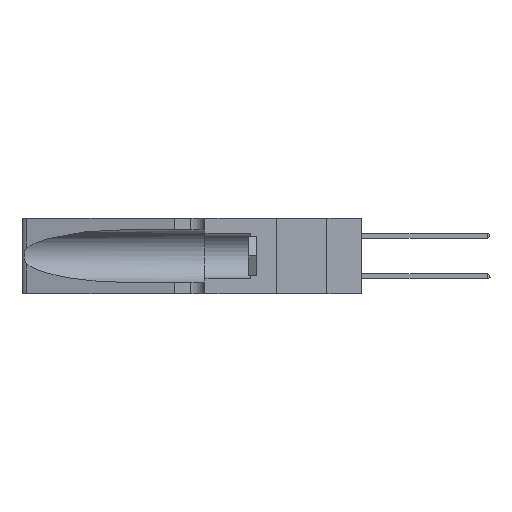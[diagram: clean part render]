
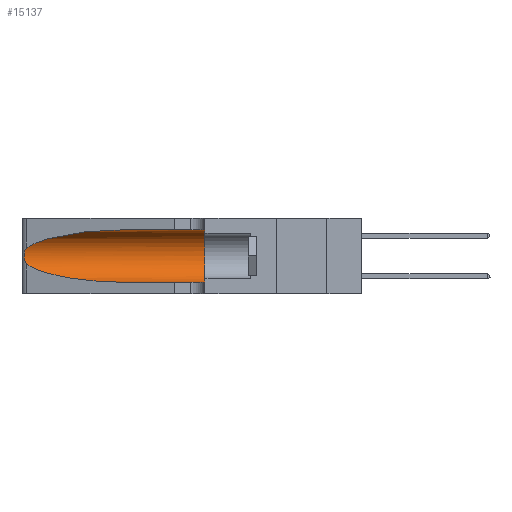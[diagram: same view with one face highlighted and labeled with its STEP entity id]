
A CAD part, left-side view. The second image highlights one B-rep face of the part: STEP entity #15137.
In plain terms, the highlighted cylindrical face has radius 3.308 mm (diameter 6.617 mm), a partial arc.
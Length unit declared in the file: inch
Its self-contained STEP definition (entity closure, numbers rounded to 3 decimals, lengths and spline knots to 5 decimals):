
#39 = CARTESIAN_POINT ( 'NONE',  ( 0.26017, 1.23833, 0.17102 ) ) ;
#55 = ORIENTED_EDGE ( 'NONE', *, *, #19286, .T. ) ;
#152 = CARTESIAN_POINT ( 'NONE',  ( 0.26075, 1.23896, 0.19203 ) ) ;
#261 = CARTESIAN_POINT ( 'NONE',  ( 0.1305, 1.61858, 0.05475 ) ) ;
#587 = CARTESIAN_POINT ( 'NONE',  ( 0.1305, 0.35, 0.185 ) ) ;
#1008 = CARTESIAN_POINT ( 'NONE',  ( 0.25487, 1.22718, 0.22369 ) ) ;
#2813 = CARTESIAN_POINT ( 'NONE',  ( 0.18966, 0.96281, 0.31525 ) ) ;
#3195 = CARTESIAN_POINT ( 'NONE',  ( 0.25639, 1.23186, 0.15144 ) ) ;
#3668 = B_SPLINE_CURVE_WITH_KNOTS ( 'NONE', 3,
 ( #23831, #9269, #23954, #18016, #5847, #26988, #152, #15075, #39, #33325, #36164, #3195, #8902, #30044 ),
 .UNSPECIFIED., .F., .F.,
 ( 4, 2, 2, 2, 2, 2, 4 ),
 ( 0., 0.00027, 0.00053, 0.00107, 0.0016, 0.00187, 0.00214 ),
 .UNSPECIFIED. ) ;
#4745 = VERTEX_POINT ( 'NONE', #27043 ) ;
#5590 = ORIENTED_EDGE ( 'NONE', *, *, #26484, .T. ) ;
#5693 = CARTESIAN_POINT ( 'NONE',  ( 0.1305, 0.72297, 0.31525 ) ) ;
#5847 = CARTESIAN_POINT ( 'NONE',  ( 0.25854, 1.2359, 0.20912 ) ) ;
#5869 =( BOUNDED_CURVE ( )  B_SPLINE_CURVE ( 3, ( #38904, #24022, #11846, #33018 ),
 .UNSPECIFIED., .F., .T. ) 
 B_SPLINE_CURVE_WITH_KNOTS ( ( 4, 4 ),
 ( 3.44316, 4.71239 ),
 .UNSPECIFIED. ) 
 CURVE ( )  GEOMETRIC_REPRESENTATION_ITEM ( )  RATIONAL_B_SPLINE_CURVE ( ( 1., 0.87, 0.87, 1. ) ) 
 REPRESENTATION_ITEM ( '' )  );
#6136 = ORIENTED_EDGE ( 'NONE', *, *, #13346, .T. ) ;
#7118 = VERTEX_POINT ( 'NONE', #35949 ) ;
#7136 = CARTESIAN_POINT ( 'NONE',  ( 0.1305, 0.72297, 0.05475 ) ) ;
#7799 = VERTEX_POINT ( 'NONE', #35772 ) ;
#8902 = CARTESIAN_POINT ( 'NONE',  ( 0.25555, 1.22993, 0.14849 ) ) ;
#9269 = CARTESIAN_POINT ( 'NONE',  ( 0.25555, 1.22994, 0.2215 ) ) ;
#10227 = EDGE_LOOP ( 'NONE', ( #5590, #55, #6136, #20827, #31502, #20986 ) ) ;
#10942 = EDGE_CURVE ( 'NONE', #19203, #4745, #27670, .T. ) ;
#10996 = VERTEX_POINT ( 'NONE', #7136 ) ;
#11846 = CARTESIAN_POINT ( 'NONE',  ( 0.18966, 0.96281, 0.05475 ) ) ;
#11889 =( BOUNDED_CURVE ( )  B_SPLINE_CURVE ( 3, ( #5693, #2813, #15047, #26830 ),
 .UNSPECIFIED., .F., .F. ) 
 B_SPLINE_CURVE_WITH_KNOTS ( ( 4, 4 ),
 ( 1.5708, 2.84003 ),
 .UNSPECIFIED. ) 
 CURVE ( )  GEOMETRIC_REPRESENTATION_ITEM ( )  RATIONAL_B_SPLINE_CURVE ( ( 1., 0.87, 0.87, 1. ) ) 
 REPRESENTATION_ITEM ( '' )  );
#12064 = VECTOR ( 'NONE', #28389, 39.37008 ) ;
#13346 = EDGE_CURVE ( 'NONE', #7118, #10996, #5869, .T. ) ;
#13672 = FACE_OUTER_BOUND ( 'NONE', #10227, .T. ) ;
#15047 = CARTESIAN_POINT ( 'NONE',  ( 0.2373, 1.15595, 0.28018 ) ) ;
#15075 = CARTESIAN_POINT ( 'NONE',  ( 0.26075, 1.23896, 0.178 ) ) ;
#15137 = ADVANCED_FACE ( 'NONE', ( #13672 ), #22686, .F. ) ;
#16101 = EDGE_CURVE ( 'NONE', #4745, #7799, #34197, .T. ) ;
#17384 = AXIS2_PLACEMENT_3D ( 'NONE', #29531, #33087, #29651 ) ;
#18016 = CARTESIAN_POINT ( 'NONE',  ( 0.25787, 1.23484, 0.2124 ) ) ;
#19203 = VERTEX_POINT ( 'NONE', #20652 ) ;
#19286 = EDGE_CURVE ( 'NONE', #27360, #7118, #3668, .T. ) ;
#20141 = EDGE_CURVE ( 'NONE', #10996, #7799, #38062, .T. ) ;
#20652 = CARTESIAN_POINT ( 'NONE',  ( 0.1305, 0.72297, 0.31525 ) ) ;
#20827 = ORIENTED_EDGE ( 'NONE', *, *, #20141, .T. ) ;
#20986 = ORIENTED_EDGE ( 'NONE', *, *, #10942, .F. ) ;
#22001 = DIRECTION ( 'NONE',  ( 0., 1., 0. ) ) ;
#22686 = CYLINDRICAL_SURFACE ( 'NONE', #17384, 0.13025 ) ;
#23824 = VECTOR ( 'NONE', #30278, 39.37008 ) ;
#23831 = CARTESIAN_POINT ( 'NONE',  ( 0.25487, 1.22718, 0.22369 ) ) ;
#23954 = CARTESIAN_POINT ( 'NONE',  ( 0.25639, 1.23184, 0.21858 ) ) ;
#24022 = CARTESIAN_POINT ( 'NONE',  ( 0.2373, 1.15595, 0.08982 ) ) ;
#24272 = AXIS2_PLACEMENT_3D ( 'NONE', #587, #22001, #36968 ) ;
#25352 = CARTESIAN_POINT ( 'NONE',  ( 0.1305, 1.61858, 0.31525 ) ) ;
#26484 = EDGE_CURVE ( 'NONE', #19203, #27360, #11889, .T. ) ;
#26830 = CARTESIAN_POINT ( 'NONE',  ( 0.25487, 1.22718, 0.22369 ) ) ;
#26988 = CARTESIAN_POINT ( 'NONE',  ( 0.26018, 1.23835, 0.19895 ) ) ;
#27043 = CARTESIAN_POINT ( 'NONE',  ( 0.1305, 0.35, 0.31525 ) ) ;
#27360 = VERTEX_POINT ( 'NONE', #1008 ) ;
#27670 = LINE ( 'NONE', #25352, #12064 ) ;
#28389 = DIRECTION ( 'NONE',  ( 0., -1., 0. ) ) ;
#29531 = CARTESIAN_POINT ( 'NONE',  ( 0.1305, 1.61858, 0.185 ) ) ;
#29651 = DIRECTION ( 'NONE',  ( 0., 0., -1. ) ) ;
#30044 = CARTESIAN_POINT ( 'NONE',  ( 0.25487, 1.22718, 0.14631 ) ) ;
#30278 = DIRECTION ( 'NONE',  ( 0., -1., 0. ) ) ;
#31502 = ORIENTED_EDGE ( 'NONE', *, *, #16101, .F. ) ;
#33018 = CARTESIAN_POINT ( 'NONE',  ( 0.1305, 0.72297, 0.05475 ) ) ;
#33087 = DIRECTION ( 'NONE',  ( 0., -1., 0. ) ) ;
#33325 = CARTESIAN_POINT ( 'NONE',  ( 0.25856, 1.23593, 0.16098 ) ) ;
#34197 = CIRCLE ( 'NONE', #24272, 0.13025 ) ;
#35772 = CARTESIAN_POINT ( 'NONE',  ( 0.1305, 0.35, 0.05475 ) ) ;
#35949 = CARTESIAN_POINT ( 'NONE',  ( 0.25487, 1.22718, 0.14631 ) ) ;
#36164 = CARTESIAN_POINT ( 'NONE',  ( 0.25789, 1.23486, 0.15765 ) ) ;
#36968 = DIRECTION ( 'NONE',  ( 0., 0., 1. ) ) ;
#38062 = LINE ( 'NONE', #261, #23824 ) ;
#38904 = CARTESIAN_POINT ( 'NONE',  ( 0.25487, 1.22718, 0.14631 ) ) ;
